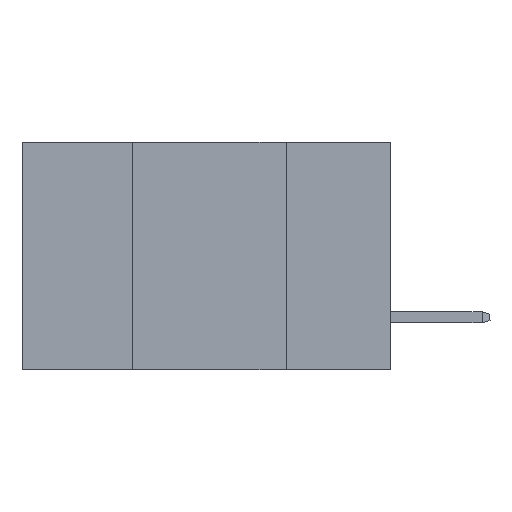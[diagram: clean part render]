
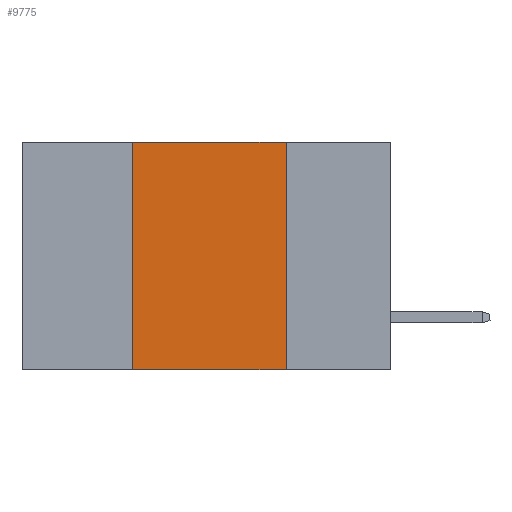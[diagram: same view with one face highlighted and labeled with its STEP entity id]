
A CAD part, left-side view. The second image highlights one B-rep face of the part: STEP entity #9775.
In plain terms, the highlighted planar face has unit normal (-1, 0, 0).
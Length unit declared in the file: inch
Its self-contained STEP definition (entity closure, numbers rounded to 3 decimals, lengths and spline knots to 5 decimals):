
#844 = PLANE ( 'NONE',  #1256 ) ;
#1015 = VERTEX_POINT ( 'NONE', #8969 ) ;
#1256 = AXIS2_PLACEMENT_3D ( 'NONE', #13748, #3065, #17942 ) ;
#1361 = VERTEX_POINT ( 'NONE', #12310 ) ;
#1738 = CARTESIAN_POINT ( 'NONE',  ( 0., 0.42, 0. ) ) ;
#1764 = CARTESIAN_POINT ( 'NONE',  ( 0., 0.6, 0. ) ) ;
#2468 = CARTESIAN_POINT ( 'NONE',  ( 0., 0.42, 0. ) ) ;
#3065 = DIRECTION ( 'NONE',  ( 1., 0., 0. ) ) ;
#4377 = EDGE_LOOP ( 'NONE', ( #14868, #26270, #5241, #19136 ) ) ;
#4650 = DIRECTION ( 'NONE',  ( 0., 0., 1. ) ) ;
#4702 = VERTEX_POINT ( 'NONE', #12540 ) ;
#5241 = ORIENTED_EDGE ( 'NONE', *, *, #6885, .F. ) ;
#5390 = LINE ( 'NONE', #1764, #16014 ) ;
#6885 = EDGE_CURVE ( 'NONE', #1361, #26360, #22333, .T. ) ;
#8771 = CARTESIAN_POINT ( 'NONE',  ( 0., 0.6, -0.37 ) ) ;
#8969 = CARTESIAN_POINT ( 'NONE',  ( 0., 0.17, 0. ) ) ;
#9096 = CARTESIAN_POINT ( 'NONE',  ( 0., 0.17, 0. ) ) ;
#9380 = VECTOR ( 'NONE', #11258, 39.37008 ) ;
#9775 = ADVANCED_FACE ( 'NONE', ( #11045 ), #844, .F. ) ;
#10320 = LINE ( 'NONE', #8771, #15198 ) ;
#10926 = DIRECTION ( 'NONE',  ( 0., -1., 0. ) ) ;
#11045 = FACE_OUTER_BOUND ( 'NONE', #4377, .T. ) ;
#11258 = DIRECTION ( 'NONE',  ( 0., 0., -1. ) ) ;
#12310 = CARTESIAN_POINT ( 'NONE',  ( 0., 0.42, -0.37 ) ) ;
#12527 = DIRECTION ( 'NONE',  ( 0., -1., 0. ) ) ;
#12540 = CARTESIAN_POINT ( 'NONE',  ( 0., 0.17, -0.37 ) ) ;
#13748 = CARTESIAN_POINT ( 'NONE',  ( 0., 0.6, 0. ) ) ;
#14868 = ORIENTED_EDGE ( 'NONE', *, *, #17168, .F. ) ;
#15198 = VECTOR ( 'NONE', #10926, 39.37008 ) ;
#15645 = EDGE_CURVE ( 'NONE', #26360, #1015, #5390, .T. ) ;
#16014 = VECTOR ( 'NONE', #12527, 39.37008 ) ;
#17168 = EDGE_CURVE ( 'NONE', #1015, #4702, #26012, .T. ) ;
#17942 = DIRECTION ( 'NONE',  ( 0., 0., -1. ) ) ;
#18211 = EDGE_CURVE ( 'NONE', #1361, #4702, #10320, .T. ) ;
#19136 = ORIENTED_EDGE ( 'NONE', *, *, #18211, .T. ) ;
#21699 = VECTOR ( 'NONE', #4650, 39.37008 ) ;
#22333 = LINE ( 'NONE', #2468, #21699 ) ;
#26012 = LINE ( 'NONE', #9096, #9380 ) ;
#26270 = ORIENTED_EDGE ( 'NONE', *, *, #15645, .F. ) ;
#26360 = VERTEX_POINT ( 'NONE', #1738 ) ;
